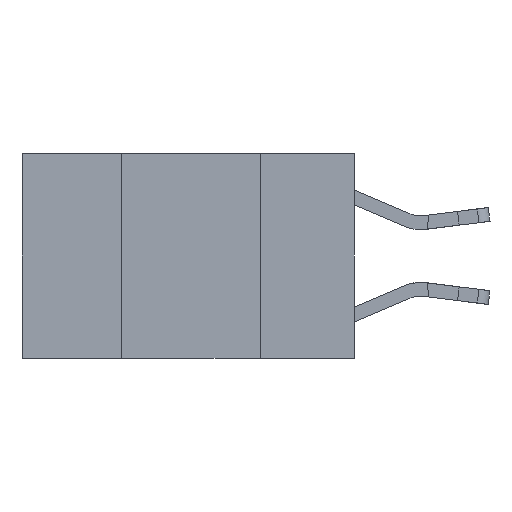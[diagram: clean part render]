
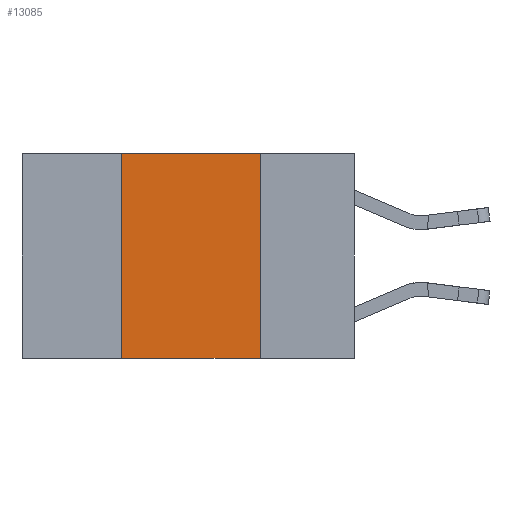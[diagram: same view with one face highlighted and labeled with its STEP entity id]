
A CAD part, left-side view. The second image highlights one B-rep face of the part: STEP entity #13085.
In plain terms, the highlighted planar face has unit normal (-1, 0, 0).
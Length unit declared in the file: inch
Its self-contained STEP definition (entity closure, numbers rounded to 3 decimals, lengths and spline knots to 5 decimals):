
#507 = CARTESIAN_POINT ( 'NONE',  ( 0., 0.6, 0. ) ) ;
#1113 = DIRECTION ( 'NONE',  ( 0., 0., -1. ) ) ;
#1374 = ORIENTED_EDGE ( 'NONE', *, *, #14490, .F. ) ;
#3128 = VECTOR ( 'NONE', #3399, 39.37008 ) ;
#3382 = DIRECTION ( 'NONE',  ( 0., -1., 0. ) ) ;
#3399 = DIRECTION ( 'NONE',  ( 0., 0., 1. ) ) ;
#4739 = VERTEX_POINT ( 'NONE', #21678 ) ;
#4875 = VECTOR ( 'NONE', #8693, 39.37008 ) ;
#4902 = CARTESIAN_POINT ( 'NONE',  ( 0., 0.42, -0.37 ) ) ;
#5773 = DIRECTION ( 'NONE',  ( 1., 0., 0. ) ) ;
#6686 = ORIENTED_EDGE ( 'NONE', *, *, #10627, .F. ) ;
#7867 = CARTESIAN_POINT ( 'NONE',  ( 0., 0.17, 0. ) ) ;
#8693 = DIRECTION ( 'NONE',  ( 0., -1., 0. ) ) ;
#10464 = CARTESIAN_POINT ( 'NONE',  ( 0., 0.6, -0.37 ) ) ;
#10627 = EDGE_CURVE ( 'NONE', #4739, #17873, #12416, .T. ) ;
#11023 = ORIENTED_EDGE ( 'NONE', *, *, #19396, .T. ) ;
#11780 = LINE ( 'NONE', #13319, #21125 ) ;
#12322 = LINE ( 'NONE', #19450, #3128 ) ;
#12416 = LINE ( 'NONE', #21428, #17972 ) ;
#12535 = EDGE_LOOP ( 'NONE', ( #1374, #6686, #13145, #11023 ) ) ;
#13085 = ADVANCED_FACE ( 'NONE', ( #14577 ), #16220, .F. ) ;
#13145 = ORIENTED_EDGE ( 'NONE', *, *, #16932, .F. ) ;
#13167 = DIRECTION ( 'NONE',  ( 0., 0., -1. ) ) ;
#13319 = CARTESIAN_POINT ( 'NONE',  ( 0., 0.17, 0. ) ) ;
#14490 = EDGE_CURVE ( 'NONE', #17873, #21884, #11780, .T. ) ;
#14577 = FACE_OUTER_BOUND ( 'NONE', #12535, .T. ) ;
#16220 = PLANE ( 'NONE',  #18505 ) ;
#16932 = EDGE_CURVE ( 'NONE', #17423, #4739, #12322, .T. ) ;
#17423 = VERTEX_POINT ( 'NONE', #4902 ) ;
#17873 = VERTEX_POINT ( 'NONE', #7867 ) ;
#17972 = VECTOR ( 'NONE', #3382, 39.37008 ) ;
#18505 = AXIS2_PLACEMENT_3D ( 'NONE', #507, #5773, #13167 ) ;
#18886 = CARTESIAN_POINT ( 'NONE',  ( 0., 0.17, -0.37 ) ) ;
#19235 = LINE ( 'NONE', #10464, #4875 ) ;
#19396 = EDGE_CURVE ( 'NONE', #17423, #21884, #19235, .T. ) ;
#19450 = CARTESIAN_POINT ( 'NONE',  ( 0., 0.42, 0. ) ) ;
#21125 = VECTOR ( 'NONE', #1113, 39.37008 ) ;
#21428 = CARTESIAN_POINT ( 'NONE',  ( 0., 0.6, 0. ) ) ;
#21678 = CARTESIAN_POINT ( 'NONE',  ( 0., 0.42, 0. ) ) ;
#21884 = VERTEX_POINT ( 'NONE', #18886 ) ;
